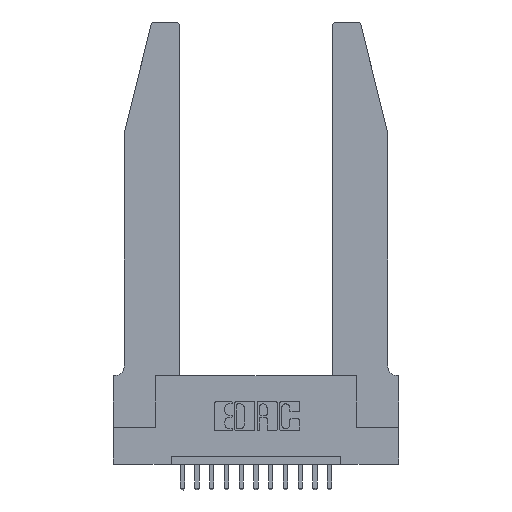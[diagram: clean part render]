
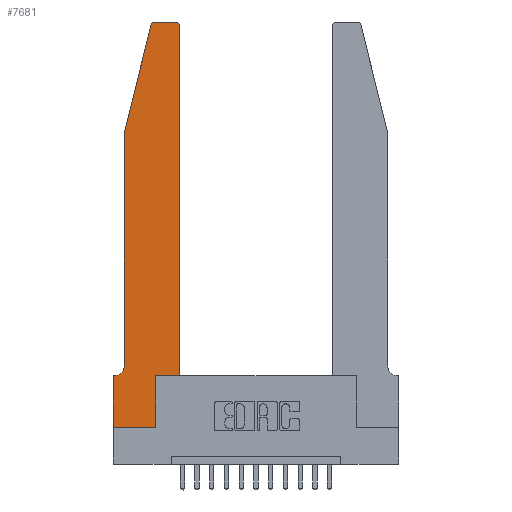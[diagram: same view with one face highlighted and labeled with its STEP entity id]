
A CAD part, top view. The second image highlights one B-rep face of the part: STEP entity #7681.
In plain terms, the highlighted planar face has unit normal (0, 0, 1).
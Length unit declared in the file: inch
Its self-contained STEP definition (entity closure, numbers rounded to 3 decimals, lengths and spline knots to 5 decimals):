
#79 = CARTESIAN_POINT ( 'NONE',  ( 0., 0.35, 0.37 ) ) ;
#131 = CARTESIAN_POINT ( 'NONE',  ( 0.0755, 2., 0.37 ) ) ;
#163 = CARTESIAN_POINT ( 'NONE',  ( 0.2865, 0.35, 0.37 ) ) ;
#418 = EDGE_CURVE ( 'NONE', #13837, #3040, #10070, .T. ) ;
#693 = LINE ( 'NONE', #6821, #8268 ) ;
#873 = VECTOR ( 'NONE', #15754, 39.37008 ) ;
#1199 = EDGE_CURVE ( 'NONE', #13006, #15625, #16926, .T. ) ;
#1237 = EDGE_CURVE ( 'NONE', #12160, #5316, #10651, .T. ) ;
#1302 = DIRECTION ( 'NONE',  ( 0., 1., 0. ) ) ;
#1376 = DIRECTION ( 'NONE',  ( 0., -1., 0. ) ) ;
#1494 = CARTESIAN_POINT ( 'NONE',  ( 0., 0.35, 0.37 ) ) ;
#1568 = VERTEX_POINT ( 'NONE', #6227 ) ;
#1662 = CARTESIAN_POINT ( 'NONE',  ( 0.284, 2.75, 0.37 ) ) ;
#1773 = DIRECTION ( 'NONE',  ( 1., 0., 0. ) ) ;
#2030 = DIRECTION ( 'NONE',  ( 1., 0., 0. ) ) ;
#2166 = EDGE_CURVE ( 'NONE', #15625, #13837, #7311, .T. ) ;
#2440 = DIRECTION ( 'NONE',  ( 0., 1., 0. ) ) ;
#2589 = VERTEX_POINT ( 'NONE', #5098 ) ;
#3040 = VERTEX_POINT ( 'NONE', #6858 ) ;
#3242 = LINE ( 'NONE', #163, #9121 ) ;
#3342 = ORIENTED_EDGE ( 'NONE', *, *, #418, .T. ) ;
#3539 = VECTOR ( 'NONE', #12094, 39.37008 ) ;
#3853 = CARTESIAN_POINT ( 'NONE',  ( 0.4205, 2.75, 0.37 ) ) ;
#3989 = LINE ( 'NONE', #5003, #873 ) ;
#4059 = DIRECTION ( 'NONE',  ( 0., 0., -1. ) ) ;
#4604 = LINE ( 'NONE', #15350, #10469 ) ;
#4726 = VECTOR ( 'NONE', #11502, 39.37008 ) ;
#4740 = EDGE_LOOP ( 'NONE', ( #12275, #14842, #10475, #3342, #15129, #12663, #10509, #9597, #15311, #16885, #7159, #10324 ) ) ;
#4834 = EDGE_CURVE ( 'NONE', #3040, #17270, #5180, .T. ) ;
#5003 = CARTESIAN_POINT ( 'NONE',  ( 0.2605, 2.75, 0.37 ) ) ;
#5098 = CARTESIAN_POINT ( 'NONE',  ( 0., 0., 0.37 ) ) ;
#5180 = CIRCLE ( 'NONE', #7573, 0.07 ) ;
#5304 = DIRECTION ( 'NONE',  ( -1., 0., 0. ) ) ;
#5316 = VERTEX_POINT ( 'NONE', #3853 ) ;
#5346 = DIRECTION ( 'NONE',  ( 0., 0., 1. ) ) ;
#5826 = EDGE_CURVE ( 'NONE', #17270, #6210, #16845, .T. ) ;
#5993 = CARTESIAN_POINT ( 'NONE',  ( 0.0055, 0.35, 0.37 ) ) ;
#6210 = VERTEX_POINT ( 'NONE', #79 ) ;
#6227 = CARTESIAN_POINT ( 'NONE',  ( 0.4505, 0.35, 0.37 ) ) ;
#6652 = CARTESIAN_POINT ( 'NONE',  ( 0.0055, 0.42, 0.37 ) ) ;
#6696 = CARTESIAN_POINT ( 'NONE',  ( 0.25487, 2.72718, 0.37 ) ) ;
#6703 = DIRECTION ( 'NONE',  ( 1., 0., 0. ) ) ;
#6821 = CARTESIAN_POINT ( 'NONE',  ( 0., 0., 0.37 ) ) ;
#6858 = CARTESIAN_POINT ( 'NONE',  ( 0.0755, 0.42, 0.37 ) ) ;
#7093 = AXIS2_PLACEMENT_3D ( 'NONE', #1494, #5346, #6703 ) ;
#7158 = LINE ( 'NONE', #16965, #7606 ) ;
#7159 = ORIENTED_EDGE ( 'NONE', *, *, #9010, .T. ) ;
#7311 = LINE ( 'NONE', #9979, #14615 ) ;
#7573 = AXIS2_PLACEMENT_3D ( 'NONE', #6652, #4059, #5304 ) ;
#7606 = VECTOR ( 'NONE', #2440, 39.37008 ) ;
#7681 = ADVANCED_FACE ( 'NONE', ( #10329 ), #8209, .T. ) ;
#7727 = CARTESIAN_POINT ( 'NONE',  ( 0.2865, 0., 0.37 ) ) ;
#8209 = PLANE ( 'NONE',  #7093 ) ;
#8268 = VECTOR ( 'NONE', #16157, 39.37008 ) ;
#8781 = DIRECTION ( 'NONE',  ( -0.239, -0.971, 0. ) ) ;
#8841 = CARTESIAN_POINT ( 'NONE',  ( 0.0755, 0.35, 0.37 ) ) ;
#8859 = CARTESIAN_POINT ( 'NONE',  ( 0.2865, 0.35, 0.37 ) ) ;
#9010 = EDGE_CURVE ( 'NONE', #1568, #12160, #7158, .T. ) ;
#9016 = EDGE_CURVE ( 'NONE', #5316, #13006, #3989, .T. ) ;
#9084 = DIRECTION ( 'NONE',  ( 0., 0., 1. ) ) ;
#9121 = VECTOR ( 'NONE', #1302, 39.37008 ) ;
#9597 = ORIENTED_EDGE ( 'NONE', *, *, #9852, .T. ) ;
#9852 = EDGE_CURVE ( 'NONE', #2589, #11735, #4604, .T. ) ;
#9905 = VERTEX_POINT ( 'NONE', #8859 ) ;
#9979 = CARTESIAN_POINT ( 'NONE',  ( 0.0755, 2., 0.37 ) ) ;
#10070 = LINE ( 'NONE', #10561, #13228 ) ;
#10246 = EDGE_CURVE ( 'NONE', #9905, #1568, #15892, .T. ) ;
#10324 = ORIENTED_EDGE ( 'NONE', *, *, #1237, .T. ) ;
#10329 = FACE_OUTER_BOUND ( 'NONE', #4740, .T. ) ;
#10469 = VECTOR ( 'NONE', #2030, 39.37008 ) ;
#10475 = ORIENTED_EDGE ( 'NONE', *, *, #2166, .T. ) ;
#10509 = ORIENTED_EDGE ( 'NONE', *, *, #14139, .T. ) ;
#10561 = CARTESIAN_POINT ( 'NONE',  ( 0.0755, 2., 0.37 ) ) ;
#10651 = CIRCLE ( 'NONE', #13252, 0.03 ) ;
#11502 = DIRECTION ( 'NONE',  ( -1., 0., 0. ) ) ;
#11735 = VERTEX_POINT ( 'NONE', #7727 ) ;
#12094 = DIRECTION ( 'NONE',  ( 1., 0., 0. ) ) ;
#12160 = VERTEX_POINT ( 'NONE', #16741 ) ;
#12275 = ORIENTED_EDGE ( 'NONE', *, *, #9016, .T. ) ;
#12441 = CARTESIAN_POINT ( 'NONE',  ( 0.284, 2.72, 0.37 ) ) ;
#12663 = ORIENTED_EDGE ( 'NONE', *, *, #5826, .T. ) ;
#12686 = EDGE_CURVE ( 'NONE', #11735, #9905, #3242, .T. ) ;
#12970 = DIRECTION ( 'NONE',  ( 1., 0., 0. ) ) ;
#13006 = VERTEX_POINT ( 'NONE', #1662 ) ;
#13025 = CARTESIAN_POINT ( 'NONE',  ( 0.4205, 2.72, 0.37 ) ) ;
#13201 = CARTESIAN_POINT ( 'NONE',  ( 0.4505, 0.35, 0.37 ) ) ;
#13228 = VECTOR ( 'NONE', #1376, 39.37008 ) ;
#13252 = AXIS2_PLACEMENT_3D ( 'NONE', #13025, #9084, #12970 ) ;
#13837 = VERTEX_POINT ( 'NONE', #131 ) ;
#14139 = EDGE_CURVE ( 'NONE', #6210, #2589, #693, .T. ) ;
#14615 = VECTOR ( 'NONE', #8781, 39.37008 ) ;
#14842 = ORIENTED_EDGE ( 'NONE', *, *, #1199, .T. ) ;
#15129 = ORIENTED_EDGE ( 'NONE', *, *, #4834, .T. ) ;
#15223 = DIRECTION ( 'NONE',  ( 0., 0., 1. ) ) ;
#15311 = ORIENTED_EDGE ( 'NONE', *, *, #12686, .T. ) ;
#15350 = CARTESIAN_POINT ( 'NONE',  ( 0., 0., 0.37 ) ) ;
#15625 = VERTEX_POINT ( 'NONE', #6696 ) ;
#15754 = DIRECTION ( 'NONE',  ( -1., 0., 0. ) ) ;
#15892 = LINE ( 'NONE', #13201, #3539 ) ;
#16157 = DIRECTION ( 'NONE',  ( 0., -1., 0. ) ) ;
#16249 = AXIS2_PLACEMENT_3D ( 'NONE', #12441, #15223, #1773 ) ;
#16741 = CARTESIAN_POINT ( 'NONE',  ( 0.4505, 2.72, 0.37 ) ) ;
#16845 = LINE ( 'NONE', #8841, #4726 ) ;
#16885 = ORIENTED_EDGE ( 'NONE', *, *, #10246, .T. ) ;
#16926 = CIRCLE ( 'NONE', #16249, 0.03 ) ;
#16965 = CARTESIAN_POINT ( 'NONE',  ( 0.4505, 0.35, 0.37 ) ) ;
#17270 = VERTEX_POINT ( 'NONE', #5993 ) ;
